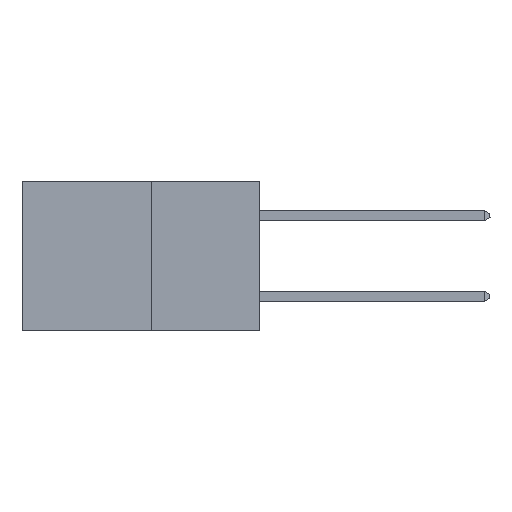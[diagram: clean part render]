
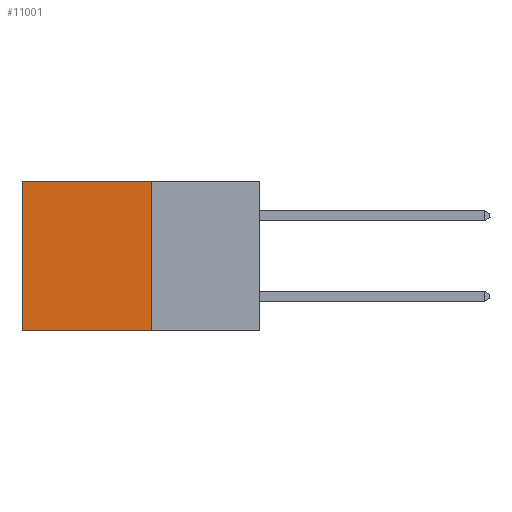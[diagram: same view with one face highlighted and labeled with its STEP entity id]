
A CAD part, left-side view. The second image highlights one B-rep face of the part: STEP entity #11001.
In plain terms, the highlighted planar face has unit normal (-1, 0, 0).
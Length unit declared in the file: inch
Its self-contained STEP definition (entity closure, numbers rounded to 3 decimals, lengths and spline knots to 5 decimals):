
#293 = DIRECTION ( 'NONE',  ( 1., 0., 0. ) ) ;
#472 = VECTOR ( 'NONE', #17822, 39.37008 ) ;
#1312 = FACE_OUTER_BOUND ( 'NONE', #12155, .T. ) ;
#1521 = DIRECTION ( 'NONE',  ( 0., 0., -1. ) ) ;
#1889 = DIRECTION ( 'NONE',  ( 0., 1., 0. ) ) ;
#2710 = CARTESIAN_POINT ( 'NONE',  ( 0.277, 0.59, 0. ) ) ;
#2734 = VERTEX_POINT ( 'NONE', #2710 ) ;
#3440 = ORIENTED_EDGE ( 'NONE', *, *, #6892, .F. ) ;
#3759 = PLANE ( 'NONE',  #6270 ) ;
#3835 = CARTESIAN_POINT ( 'NONE',  ( 0.277, 0.27, -0.37 ) ) ;
#4296 = LINE ( 'NONE', #11936, #12949 ) ;
#4556 = VECTOR ( 'NONE', #15921, 39.37008 ) ;
#4621 = VECTOR ( 'NONE', #1889, 39.37008 ) ;
#5244 = CARTESIAN_POINT ( 'NONE',  ( 0.277, 0.27, -0.37 ) ) ;
#5597 = CARTESIAN_POINT ( 'NONE',  ( 0.277, 0.59, -0.37 ) ) ;
#5777 = EDGE_CURVE ( 'NONE', #18951, #2734, #8130, .T. ) ;
#6270 = AXIS2_PLACEMENT_3D ( 'NONE', #7245, #293, #12460 ) ;
#6892 = EDGE_CURVE ( 'NONE', #18951, #12197, #4296, .T. ) ;
#7086 = EDGE_CURVE ( 'NONE', #12197, #21655, #22392, .T. ) ;
#7245 = CARTESIAN_POINT ( 'NONE',  ( 0.277, 0.27, -0.37 ) ) ;
#8050 = ORIENTED_EDGE ( 'NONE', *, *, #5777, .T. ) ;
#8130 = LINE ( 'NONE', #10537, #4621 ) ;
#9238 = CARTESIAN_POINT ( 'NONE',  ( 0.277, 0.59, -0.37 ) ) ;
#10537 = CARTESIAN_POINT ( 'NONE',  ( 0.277, 0.27, 0. ) ) ;
#11001 = ADVANCED_FACE ( 'NONE', ( #1312 ), #3759, .F. ) ;
#11715 = EDGE_CURVE ( 'NONE', #2734, #21655, #18332, .T. ) ;
#11936 = CARTESIAN_POINT ( 'NONE',  ( 0.277, 0.27, -0.37 ) ) ;
#12155 = EDGE_LOOP ( 'NONE', ( #15416, #14252, #3440, #8050 ) ) ;
#12197 = VERTEX_POINT ( 'NONE', #5244 ) ;
#12460 = DIRECTION ( 'NONE',  ( 0., 0., -1. ) ) ;
#12949 = VECTOR ( 'NONE', #1521, 39.37008 ) ;
#14252 = ORIENTED_EDGE ( 'NONE', *, *, #7086, .F. ) ;
#15416 = ORIENTED_EDGE ( 'NONE', *, *, #11715, .T. ) ;
#15921 = DIRECTION ( 'NONE',  ( 0., 1., 0. ) ) ;
#17822 = DIRECTION ( 'NONE',  ( 0., 0., -1. ) ) ;
#18332 = LINE ( 'NONE', #9238, #472 ) ;
#18951 = VERTEX_POINT ( 'NONE', #19166 ) ;
#19166 = CARTESIAN_POINT ( 'NONE',  ( 0.277, 0.27, 0. ) ) ;
#21655 = VERTEX_POINT ( 'NONE', #5597 ) ;
#22392 = LINE ( 'NONE', #3835, #4556 ) ;
